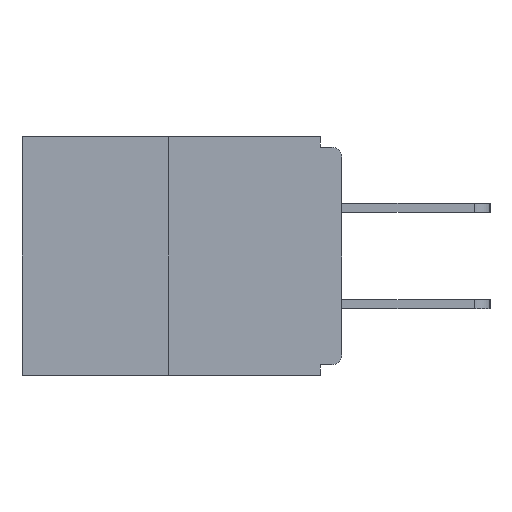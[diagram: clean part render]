
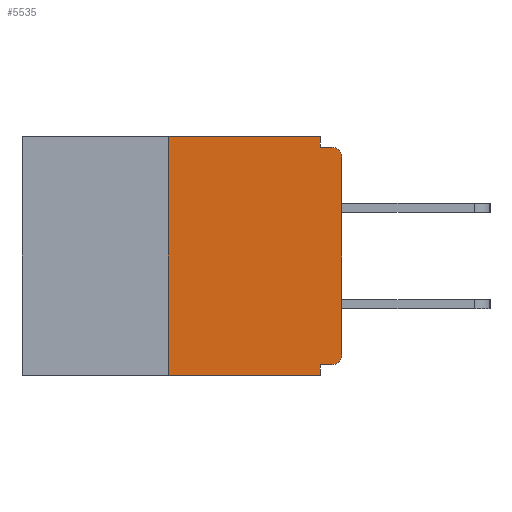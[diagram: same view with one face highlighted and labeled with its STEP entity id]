
A CAD part, left-side view. The second image highlights one B-rep face of the part: STEP entity #5535.
In plain terms, the highlighted planar face has unit normal (-1, 0, 0).
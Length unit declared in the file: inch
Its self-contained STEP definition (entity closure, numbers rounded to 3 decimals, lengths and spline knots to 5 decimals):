
#195 = CARTESIAN_POINT ( 'NONE',  ( 0., 0., -0.015 ) ) ;
#509 = CARTESIAN_POINT ( 'NONE',  ( 0., 0.031, 0. ) ) ;
#1096 = DIRECTION ( 'NONE',  ( 1., 0., 0. ) ) ;
#1180 = VERTEX_POINT ( 'NONE', #14599 ) ;
#1213 = EDGE_CURVE ( 'NONE', #12099, #6444, #5787, .T. ) ;
#1238 = CARTESIAN_POINT ( 'NONE',  ( 0., 0.031, -0.328 ) ) ;
#1255 = VERTEX_POINT ( 'NONE', #1238 ) ;
#1277 = EDGE_CURVE ( 'NONE', #4218, #12099, #12762, .T. ) ;
#1384 = VECTOR ( 'NONE', #7448, 39.37008 ) ;
#1536 = ORIENTED_EDGE ( 'NONE', *, *, #1277, .F. ) ;
#1565 = CARTESIAN_POINT ( 'NONE',  ( 0., 0.015, -0.313 ) ) ;
#1566 = ORIENTED_EDGE ( 'NONE', *, *, #13805, .F. ) ;
#1781 = EDGE_CURVE ( 'NONE', #10921, #1180, #9952, .T. ) ;
#1827 = LINE ( 'NONE', #14806, #2718 ) ;
#1958 = AXIS2_PLACEMENT_3D ( 'NONE', #1565, #9580, #11724 ) ;
#2076 = ORIENTED_EDGE ( 'NONE', *, *, #3349, .F. ) ;
#2149 = DIRECTION ( 'NONE',  ( 0., 0., 1. ) ) ;
#2282 = FACE_OUTER_BOUND ( 'NONE', #8865, .T. ) ;
#2323 = DIRECTION ( 'NONE',  ( 0., 0., 1. ) ) ;
#2718 = VECTOR ( 'NONE', #10217, 39.37008 ) ;
#2903 = LINE ( 'NONE', #195, #4320 ) ;
#3349 = EDGE_CURVE ( 'NONE', #1255, #8607, #1827, .T. ) ;
#3436 = LINE ( 'NONE', #509, #9865 ) ;
#3561 = DIRECTION ( 'NONE',  ( 0., -1., 0. ) ) ;
#3672 = VECTOR ( 'NONE', #2149, 39.37008 ) ;
#3896 = DIRECTION ( 'NONE',  ( 0., 0., -1. ) ) ;
#3967 = ORIENTED_EDGE ( 'NONE', *, *, #1213, .F. ) ;
#4216 = ORIENTED_EDGE ( 'NONE', *, *, #5824, .T. ) ;
#4218 = VERTEX_POINT ( 'NONE', #4527 ) ;
#4284 = CARTESIAN_POINT ( 'NONE',  ( 0., 0., -0.03 ) ) ;
#4320 = VECTOR ( 'NONE', #3561, 39.37008 ) ;
#4413 = VECTOR ( 'NONE', #7177, 39.37008 ) ;
#4420 = CARTESIAN_POINT ( 'NONE',  ( 0., 0.46, 0. ) ) ;
#4518 = DIRECTION ( 'NONE',  ( 0., -1., 0. ) ) ;
#4527 = CARTESIAN_POINT ( 'NONE',  ( 0., 0.25, -0.343 ) ) ;
#4586 = ORIENTED_EDGE ( 'NONE', *, *, #13019, .T. ) ;
#5151 = CARTESIAN_POINT ( 'NONE',  ( 0., 0.015, -0.03 ) ) ;
#5531 = VERTEX_POINT ( 'NONE', #10115 ) ;
#5535 = ADVANCED_FACE ( 'NONE', ( #2282 ), #11329, .F. ) ;
#5688 = DIRECTION ( 'NONE',  ( 0., 0., -1. ) ) ;
#5720 = EDGE_CURVE ( 'NONE', #5887, #1255, #6587, .T. ) ;
#5787 = LINE ( 'NONE', #4420, #14741 ) ;
#5824 = EDGE_CURVE ( 'NONE', #4218, #8607, #8920, .T. ) ;
#5887 = VERTEX_POINT ( 'NONE', #7216 ) ;
#6122 = CIRCLE ( 'NONE', #1958, 0.015 ) ;
#6146 = CARTESIAN_POINT ( 'NONE',  ( 0., 0., -0.313 ) ) ;
#6162 = CARTESIAN_POINT ( 'NONE',  ( 0., 0.25, 0. ) ) ;
#6335 = CARTESIAN_POINT ( 'NONE',  ( 0., 0.46, -0.343 ) ) ;
#6444 = VERTEX_POINT ( 'NONE', #10850 ) ;
#6587 = LINE ( 'NONE', #14092, #4413 ) ;
#6655 = CARTESIAN_POINT ( 'NONE',  ( 0., 0., 0. ) ) ;
#6849 = CARTESIAN_POINT ( 'NONE',  ( 0., 0.031, -0.343 ) ) ;
#7019 = AXIS2_PLACEMENT_3D ( 'NONE', #5151, #10769, #8500 ) ;
#7177 = DIRECTION ( 'NONE',  ( 0., 1., 0. ) ) ;
#7216 = CARTESIAN_POINT ( 'NONE',  ( 0., 0.015, -0.328 ) ) ;
#7233 = ORIENTED_EDGE ( 'NONE', *, *, #8436, .F. ) ;
#7448 = DIRECTION ( 'NONE',  ( 0., -1., 0. ) ) ;
#8007 = ORIENTED_EDGE ( 'NONE', *, *, #8052, .T. ) ;
#8052 = EDGE_CURVE ( 'NONE', #5887, #10698, #6122, .T. ) ;
#8436 = EDGE_CURVE ( 'NONE', #5531, #1180, #2903, .T. ) ;
#8500 = DIRECTION ( 'NONE',  ( 0., 0., -1. ) ) ;
#8607 = VERTEX_POINT ( 'NONE', #6849 ) ;
#8865 = EDGE_LOOP ( 'NONE', ( #3967, #1536, #4216, #2076, #14141, #8007, #4586, #12176, #7233, #1566 ) ) ;
#8920 = LINE ( 'NONE', #6335, #1384 ) ;
#9580 = DIRECTION ( 'NONE',  ( -1., 0., 0. ) ) ;
#9865 = VECTOR ( 'NONE', #3896, 39.37008 ) ;
#9952 = CIRCLE ( 'NONE', #7019, 0.015 ) ;
#10115 = CARTESIAN_POINT ( 'NONE',  ( 0., 0.031, -0.015 ) ) ;
#10217 = DIRECTION ( 'NONE',  ( 0., 0., -1. ) ) ;
#10698 = VERTEX_POINT ( 'NONE', #6146 ) ;
#10769 = DIRECTION ( 'NONE',  ( -1., 0., 0. ) ) ;
#10850 = CARTESIAN_POINT ( 'NONE',  ( 0., 0.031, 0. ) ) ;
#10921 = VERTEX_POINT ( 'NONE', #4284 ) ;
#11329 = PLANE ( 'NONE',  #12201 ) ;
#11724 = DIRECTION ( 'NONE',  ( 0., 0., -1. ) ) ;
#12099 = VERTEX_POINT ( 'NONE', #6162 ) ;
#12176 = ORIENTED_EDGE ( 'NONE', *, *, #1781, .T. ) ;
#12201 = AXIS2_PLACEMENT_3D ( 'NONE', #13544, #1096, #5688 ) ;
#12406 = VECTOR ( 'NONE', #2323, 39.37008 ) ;
#12762 = LINE ( 'NONE', #13682, #12406 ) ;
#12804 = LINE ( 'NONE', #6655, #3672 ) ;
#13019 = EDGE_CURVE ( 'NONE', #10698, #10921, #12804, .T. ) ;
#13544 = CARTESIAN_POINT ( 'NONE',  ( 0., 0.46, 0. ) ) ;
#13682 = CARTESIAN_POINT ( 'NONE',  ( 0., 0.25, 0. ) ) ;
#13805 = EDGE_CURVE ( 'NONE', #6444, #5531, #3436, .T. ) ;
#14092 = CARTESIAN_POINT ( 'NONE',  ( 0., 0., -0.328 ) ) ;
#14141 = ORIENTED_EDGE ( 'NONE', *, *, #5720, .F. ) ;
#14599 = CARTESIAN_POINT ( 'NONE',  ( 0., 0.015, -0.015 ) ) ;
#14741 = VECTOR ( 'NONE', #4518, 39.37008 ) ;
#14806 = CARTESIAN_POINT ( 'NONE',  ( 0., 0.031, -0.343 ) ) ;
